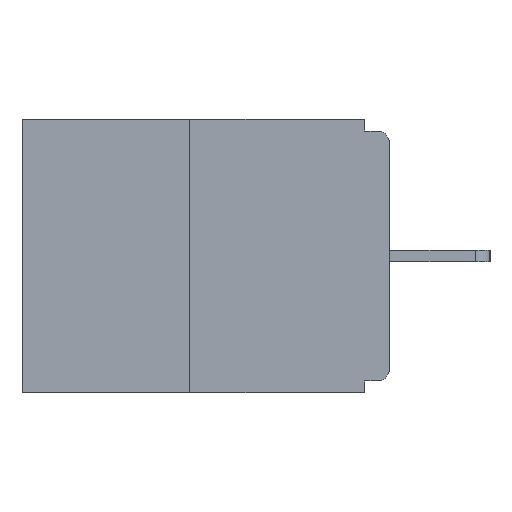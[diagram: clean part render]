
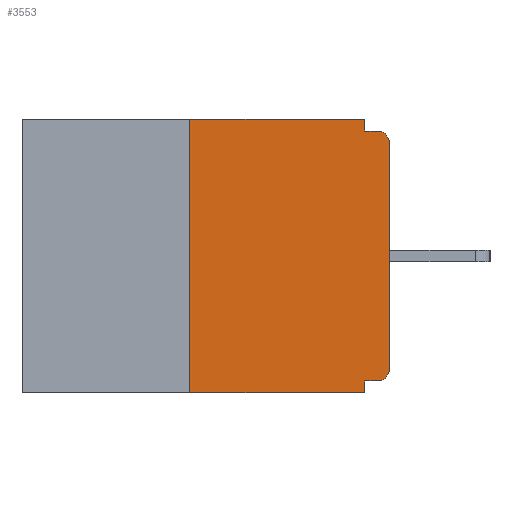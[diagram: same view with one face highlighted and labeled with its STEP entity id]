
A CAD part, left-side view. The second image highlights one B-rep face of the part: STEP entity #3553.
In plain terms, the highlighted planar face has unit normal (-1, 0, 0).
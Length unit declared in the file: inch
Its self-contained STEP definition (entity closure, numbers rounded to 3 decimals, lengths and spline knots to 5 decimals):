
#198 = AXIS2_PLACEMENT_3D ( 'NONE', #5150, #5087, #9415 ) ;
#348 = EDGE_CURVE ( 'NONE', #13004, #4237, #11795, .T. ) ;
#719 = EDGE_CURVE ( 'NONE', #12366, #7610, #7167, .T. ) ;
#892 = VECTOR ( 'NONE', #7032, 39.37008 ) ;
#917 = DIRECTION ( 'NONE',  ( 0., 0., -1. ) ) ;
#951 = ORIENTED_EDGE ( 'NONE', *, *, #5192, .F. ) ;
#1636 = VERTEX_POINT ( 'NONE', #2632 ) ;
#1811 = CARTESIAN_POINT ( 'NONE',  ( 0., 0.031, -0.328 ) ) ;
#1891 = ORIENTED_EDGE ( 'NONE', *, *, #10261, .T. ) ;
#1966 = EDGE_CURVE ( 'NONE', #8047, #6427, #4873, .T. ) ;
#1996 = DIRECTION ( 'NONE',  ( 1., 0., 0. ) ) ;
#2152 = CIRCLE ( 'NONE', #7521, 0.015 ) ;
#2544 = VECTOR ( 'NONE', #2895, 39.37008 ) ;
#2632 = CARTESIAN_POINT ( 'NONE',  ( 0., 0.031, -0.015 ) ) ;
#2697 = CARTESIAN_POINT ( 'NONE',  ( 0., 0.25, 0. ) ) ;
#2713 = ORIENTED_EDGE ( 'NONE', *, *, #719, .T. ) ;
#2865 = ORIENTED_EDGE ( 'NONE', *, *, #11203, .F. ) ;
#2895 = DIRECTION ( 'NONE',  ( 0., 0., 1. ) ) ;
#3028 = CARTESIAN_POINT ( 'NONE',  ( 0., 0.031, 0. ) ) ;
#3039 = PLANE ( 'NONE',  #3110 ) ;
#3110 = AXIS2_PLACEMENT_3D ( 'NONE', #7320, #1996, #6267 ) ;
#3505 = CARTESIAN_POINT ( 'NONE',  ( 0., 0.25, -0.343 ) ) ;
#3551 = EDGE_CURVE ( 'NONE', #9179, #11810, #8713, .T. ) ;
#3553 = ADVANCED_FACE ( 'NONE', ( #12629 ), #3039, .F. ) ;
#3552 = VECTOR ( 'NONE', #9072, 39.37008 ) ;
#3663 = ORIENTED_EDGE ( 'NONE', *, *, #5869, .T. ) ;
#4179 = CARTESIAN_POINT ( 'NONE',  ( 0., 0.031, -0.343 ) ) ;
#4237 = VERTEX_POINT ( 'NONE', #1811 ) ;
#4261 = VECTOR ( 'NONE', #8582, 39.37008 ) ;
#4873 = LINE ( 'NONE', #9145, #892 ) ;
#5087 = DIRECTION ( 'NONE',  ( -1., 0., 0. ) ) ;
#5150 = CARTESIAN_POINT ( 'NONE',  ( 0., 0.015, -0.03 ) ) ;
#5192 = EDGE_CURVE ( 'NONE', #4237, #7610, #7736, .T. ) ;
#5366 = CARTESIAN_POINT ( 'NONE',  ( 0., 0.015, -0.328 ) ) ;
#5869 = EDGE_CURVE ( 'NONE', #7390, #9179, #7135, .T. ) ;
#5874 = VECTOR ( 'NONE', #10996, 39.37008 ) ;
#6060 = CARTESIAN_POINT ( 'NONE',  ( 0., 0.46, -0.343 ) ) ;
#6091 = DIRECTION ( 'NONE',  ( 0., -1., 0. ) ) ;
#6179 = EDGE_CURVE ( 'NONE', #12366, #8047, #10104, .T. ) ;
#6267 = DIRECTION ( 'NONE',  ( 0., 0., -1. ) ) ;
#6427 = VERTEX_POINT ( 'NONE', #9670 ) ;
#6725 = CARTESIAN_POINT ( 'NONE',  ( 0., 0.031, -0.343 ) ) ;
#7032 = DIRECTION ( 'NONE',  ( 0., -1., 0. ) ) ;
#7135 = LINE ( 'NONE', #11529, #12581 ) ;
#7167 = LINE ( 'NONE', #6060, #3552 ) ;
#7320 = CARTESIAN_POINT ( 'NONE',  ( 0., 0.46, 0. ) ) ;
#7390 = VERTEX_POINT ( 'NONE', #9600 ) ;
#7410 = ORIENTED_EDGE ( 'NONE', *, *, #348, .F. ) ;
#7448 = VECTOR ( 'NONE', #6091, 39.37008 ) ;
#7521 = AXIS2_PLACEMENT_3D ( 'NONE', #10981, #9651, #9728 ) ;
#7610 = VERTEX_POINT ( 'NONE', #4179 ) ;
#7736 = LINE ( 'NONE', #6725, #5874 ) ;
#8047 = VERTEX_POINT ( 'NONE', #8244 ) ;
#8244 = CARTESIAN_POINT ( 'NONE',  ( 0., 0.25, 0. ) ) ;
#8530 = ORIENTED_EDGE ( 'NONE', *, *, #6179, .F. ) ;
#8582 = DIRECTION ( 'NONE',  ( 0., 1., 0. ) ) ;
#8713 = CIRCLE ( 'NONE', #198, 0.015 ) ;
#8929 = ORIENTED_EDGE ( 'NONE', *, *, #9757, .F. ) ;
#9072 = DIRECTION ( 'NONE',  ( 0., -1., 0. ) ) ;
#9145 = CARTESIAN_POINT ( 'NONE',  ( 0., 0.46, 0. ) ) ;
#9179 = VERTEX_POINT ( 'NONE', #12102 ) ;
#9415 = DIRECTION ( 'NONE',  ( 0., 0., -1. ) ) ;
#9571 = EDGE_LOOP ( 'NONE', ( #11815, #8530, #2713, #951, #7410, #1891, #3663, #10376, #2865, #8929 ) ) ;
#9600 = CARTESIAN_POINT ( 'NONE',  ( 0., 0., -0.313 ) ) ;
#9651 = DIRECTION ( 'NONE',  ( -1., 0., 0. ) ) ;
#9670 = CARTESIAN_POINT ( 'NONE',  ( 0., 0.031, 0. ) ) ;
#9728 = DIRECTION ( 'NONE',  ( 0., 0., -1. ) ) ;
#9757 = EDGE_CURVE ( 'NONE', #6427, #1636, #10652, .T. ) ;
#9820 = CARTESIAN_POINT ( 'NONE',  ( 0., 0.015, -0.015 ) ) ;
#10104 = LINE ( 'NONE', #2697, #2544 ) ;
#10261 = EDGE_CURVE ( 'NONE', #13004, #7390, #2152, .T. ) ;
#10376 = ORIENTED_EDGE ( 'NONE', *, *, #3551, .T. ) ;
#10470 = CARTESIAN_POINT ( 'NONE',  ( 0., 0., -0.328 ) ) ;
#10652 = LINE ( 'NONE', #3028, #12424 ) ;
#10981 = CARTESIAN_POINT ( 'NONE',  ( 0., 0.015, -0.313 ) ) ;
#10996 = DIRECTION ( 'NONE',  ( 0., 0., -1. ) ) ;
#11203 = EDGE_CURVE ( 'NONE', #1636, #11810, #11725, .T. ) ;
#11529 = CARTESIAN_POINT ( 'NONE',  ( 0., 0., 0. ) ) ;
#11725 = LINE ( 'NONE', #13437, #7448 ) ;
#11795 = LINE ( 'NONE', #10470, #4261 ) ;
#11810 = VERTEX_POINT ( 'NONE', #9820 ) ;
#11815 = ORIENTED_EDGE ( 'NONE', *, *, #1966, .F. ) ;
#12102 = CARTESIAN_POINT ( 'NONE',  ( 0., 0., -0.03 ) ) ;
#12366 = VERTEX_POINT ( 'NONE', #3505 ) ;
#12424 = VECTOR ( 'NONE', #917, 39.37008 ) ;
#12514 = DIRECTION ( 'NONE',  ( 0., 0., 1. ) ) ;
#12581 = VECTOR ( 'NONE', #12514, 39.37008 ) ;
#12629 = FACE_OUTER_BOUND ( 'NONE', #9571, .T. ) ;
#13004 = VERTEX_POINT ( 'NONE', #5366 ) ;
#13437 = CARTESIAN_POINT ( 'NONE',  ( 0., 0., -0.015 ) ) ;
